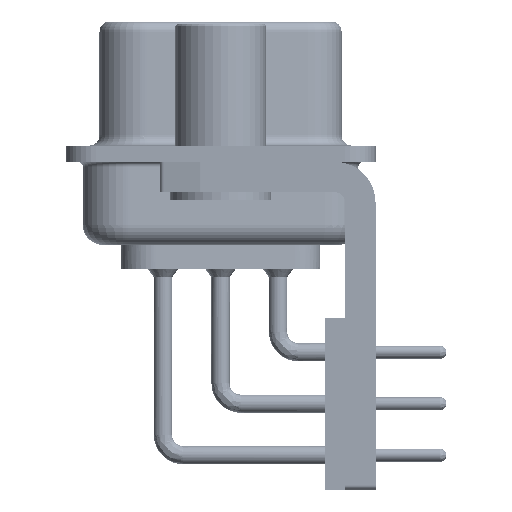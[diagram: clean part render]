
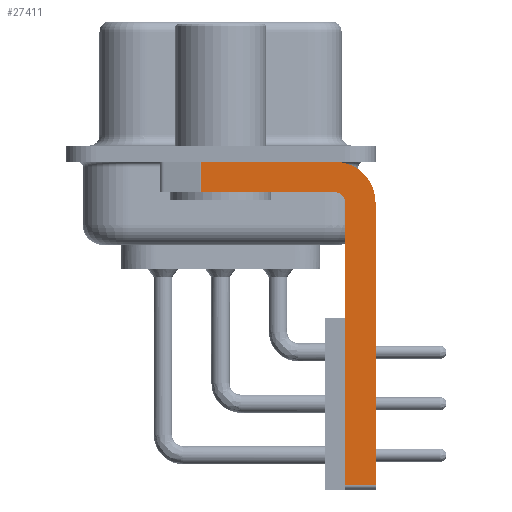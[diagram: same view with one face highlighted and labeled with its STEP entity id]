
A CAD part, left-side view. The second image highlights one B-rep face of the part: STEP entity #27411.
In plain terms, the highlighted planar face has unit normal (-1, 0, 0).
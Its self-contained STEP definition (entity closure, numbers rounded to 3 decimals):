
#178 = CARTESIAN_POINT ( 'NONE',  ( -2.9, -5.65, -2.4 ) ) ;
#655 = CARTESIAN_POINT ( 'NONE',  ( -2.9, -5.65, -0.4 ) ) ;
#2278 = CARTESIAN_POINT ( 'NONE',  ( -2.9, -5.65, -16.35 ) ) ;
#3540 = DIRECTION ( 'NONE',  ( 0., 0., -1. ) ) ;
#3841 = VECTOR ( 'NONE', #12194, 1000. ) ;
#5777 = ORIENTED_EDGE ( 'NONE', *, *, #38592, .F. ) ;
#5803 = DIRECTION ( 'NONE',  ( -1., 0., 0. ) ) ;
#6037 = DIRECTION ( 'NONE',  ( 0., 0., -1. ) ) ;
#7610 = ORIENTED_EDGE ( 'NONE', *, *, #36202, .T. ) ;
#8564 = DIRECTION ( 'NONE',  ( 0., 0., -1. ) ) ;
#8860 = VERTEX_POINT ( 'NONE', #12486 ) ;
#8868 = CARTESIAN_POINT ( 'NONE',  ( -2.9, -6.15, -16.6 ) ) ;
#9235 = CARTESIAN_POINT ( 'NONE',  ( -2.9, -7.65, -2.4 ) ) ;
#9439 = CARTESIAN_POINT ( 'NONE',  ( -2.9, 0.978, -0.4 ) ) ;
#9585 = AXIS2_PLACEMENT_3D ( 'NONE', #178, #23525, #3540 ) ;
#9596 = ORIENTED_EDGE ( 'NONE', *, *, #24533, .F. ) ;
#10686 = VECTOR ( 'NONE', #42874, 1000. ) ;
#11616 = PLANE ( 'NONE',  #32445 ) ;
#11757 = CARTESIAN_POINT ( 'NONE',  ( -2.9, -5.65, -2.4 ) ) ;
#12152 = CARTESIAN_POINT ( 'NONE',  ( -2.9, -5.65, -1.9 ) ) ;
#12194 = DIRECTION ( 'NONE',  ( 0., 0., 1. ) ) ;
#12486 = CARTESIAN_POINT ( 'NONE',  ( -2.9, -7.65, -2.4 ) ) ;
#12944 = CIRCLE ( 'NONE', #9585, 2. ) ;
#12964 = VECTOR ( 'NONE', #6037, 1000. ) ;
#13053 = VERTEX_POINT ( 'NONE', #23210 ) ;
#13094 = CARTESIAN_POINT ( 'NONE',  ( -2.9, 0.978, -1.9 ) ) ;
#13272 = ORIENTED_EDGE ( 'NONE', *, *, #18289, .F. ) ;
#13486 = EDGE_CURVE ( 'NONE', #32791, #21771, #24303, .T. ) ;
#15056 = LINE ( 'NONE', #9235, #12964 ) ;
#15100 = VERTEX_POINT ( 'NONE', #21276 ) ;
#15452 = CARTESIAN_POINT ( 'NONE',  ( -2.9, -6.15, -2.4 ) ) ;
#17351 = EDGE_CURVE ( 'NONE', #27595, #33724, #17906, .T. ) ;
#17906 = LINE ( 'NONE', #41006, #26753 ) ;
#18289 = EDGE_CURVE ( 'NONE', #15100, #32791, #30375, .T. ) ;
#19385 = ORIENTED_EDGE ( 'NONE', *, *, #42431, .F. ) ;
#19579 = LINE ( 'NONE', #36155, #10686 ) ;
#21276 = CARTESIAN_POINT ( 'NONE',  ( -2.9, -6.15, -16.35 ) ) ;
#21771 = VERTEX_POINT ( 'NONE', #12152 ) ;
#22263 = DIRECTION ( 'NONE',  ( 0., -1., 0. ) ) ;
#22903 = ORIENTED_EDGE ( 'NONE', *, *, #13486, .F. ) ;
#23210 = CARTESIAN_POINT ( 'NONE',  ( -2.9, -7.65, -16.35 ) ) ;
#23525 = DIRECTION ( 'NONE',  ( 1., 0., 0. ) ) ;
#24303 = CIRCLE ( 'NONE', #39843, 0.5 ) ;
#24488 = VECTOR ( 'NONE', #22263, 1000. ) ;
#24533 = EDGE_CURVE ( 'NONE', #8860, #13053, #15056, .T. ) ;
#25173 = VECTOR ( 'NONE', #41961, 1000. ) ;
#25520 = LINE ( 'NONE', #2278, #24488 ) ;
#25729 = CARTESIAN_POINT ( 'NONE',  ( -2.9, -5.65, -2.4 ) ) ;
#26753 = VECTOR ( 'NONE', #27544, 1000. ) ;
#27411 = ADVANCED_FACE ( 'NONE', ( #29354 ), #11616, .F. ) ;
#27544 = DIRECTION ( 'NONE',  ( 0., -1., 0. ) ) ;
#27595 = VERTEX_POINT ( 'NONE', #9439 ) ;
#28481 = DIRECTION ( 'NONE',  ( 1., 0., 0. ) ) ;
#29045 = DIRECTION ( 'NONE',  ( 0., 0., 1. ) ) ;
#29354 = FACE_OUTER_BOUND ( 'NONE', #41973, .T. ) ;
#30375 = LINE ( 'NONE', #8868, #3841 ) ;
#31445 = ORIENTED_EDGE ( 'NONE', *, *, #17351, .F. ) ;
#32445 = AXIS2_PLACEMENT_3D ( 'NONE', #11757, #28481, #8564 ) ;
#32791 = VERTEX_POINT ( 'NONE', #15452 ) ;
#33386 = EDGE_CURVE ( 'NONE', #15100, #13053, #25520, .T. ) ;
#33724 = VERTEX_POINT ( 'NONE', #655 ) ;
#34051 = LINE ( 'NONE', #38759, #25173 ) ;
#36155 = CARTESIAN_POINT ( 'NONE',  ( -2.9, 0.978, -1.9 ) ) ;
#36202 = EDGE_CURVE ( 'NONE', #27595, #36930, #19579, .T. ) ;
#36930 = VERTEX_POINT ( 'NONE', #13094 ) ;
#38592 = EDGE_CURVE ( 'NONE', #21771, #36930, #34051, .T. ) ;
#38759 = CARTESIAN_POINT ( 'NONE',  ( -2.9, -5.65, -1.9 ) ) ;
#39843 = AXIS2_PLACEMENT_3D ( 'NONE', #25729, #5803, #29045 ) ;
#41006 = CARTESIAN_POINT ( 'NONE',  ( -2.9, 3., -0.4 ) ) ;
#41961 = DIRECTION ( 'NONE',  ( 0., 1., 0. ) ) ;
#41973 = EDGE_LOOP ( 'NONE', ( #31445, #7610, #5777, #22903, #13272, #42298, #9596, #19385 ) ) ;
#42298 = ORIENTED_EDGE ( 'NONE', *, *, #33386, .T. ) ;
#42431 = EDGE_CURVE ( 'NONE', #33724, #8860, #12944, .T. ) ;
#42874 = DIRECTION ( 'NONE',  ( 0., 0., -1. ) ) ;
